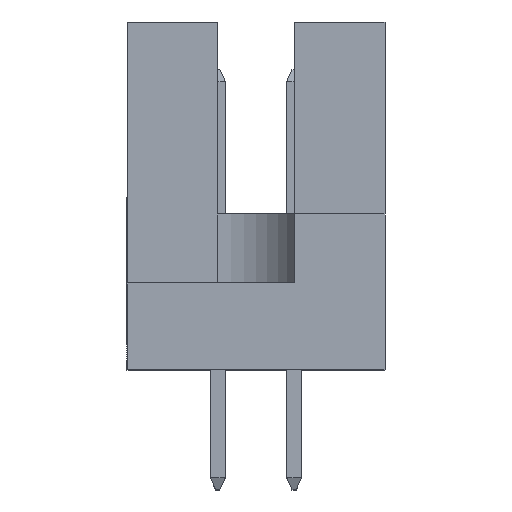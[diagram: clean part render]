
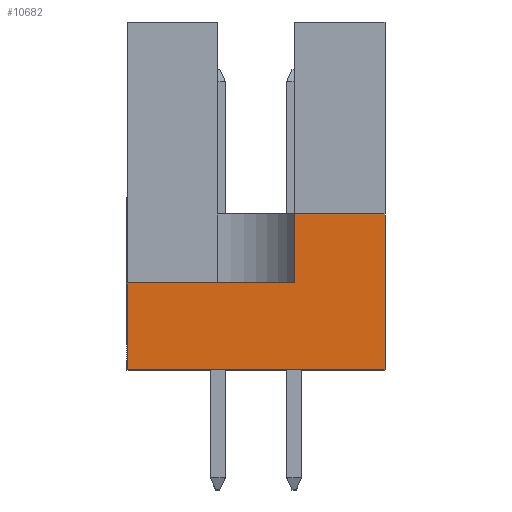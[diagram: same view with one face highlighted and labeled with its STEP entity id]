
A CAD part, left-side view. The second image highlights one B-rep face of the part: STEP entity #10682.
In plain terms, the highlighted planar face has unit normal (-1, 0, 0).
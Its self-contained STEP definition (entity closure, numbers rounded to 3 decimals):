
#444 = EDGE_CURVE ( 'NONE', #10742, #10309, #2380, .T. ) ;
#518 = VERTEX_POINT ( 'NONE', #10656 ) ;
#598 = FACE_OUTER_BOUND ( 'NONE', #5916, .T. ) ;
#908 = DIRECTION ( 'NONE',  ( 0., 0., -1. ) ) ;
#1095 = ORIENTED_EDGE ( 'NONE', *, *, #4684, .F. ) ;
#1293 = DIRECTION ( 'NONE',  ( 0., 0., -1. ) ) ;
#1471 = DIRECTION ( 'NONE',  ( 0., -1., 0. ) ) ;
#2091 = CARTESIAN_POINT ( 'NONE',  ( -47.5, 4.3, 11.6 ) ) ;
#2115 = CARTESIAN_POINT ( 'NONE',  ( -47.5, 4.3, 2.9 ) ) ;
#2380 = LINE ( 'NONE', #10337, #5114 ) ;
#2808 = VECTOR ( 'NONE', #3767, 1000. ) ;
#3012 = DIRECTION ( 'NONE',  ( 1., 0., 0. ) ) ;
#3063 = CARTESIAN_POINT ( 'NONE',  ( -47.5, 4.3, 11.6 ) ) ;
#3296 = ORIENTED_EDGE ( 'NONE', *, *, #444, .F. ) ;
#3382 = VECTOR ( 'NONE', #908, 1000. ) ;
#3767 = DIRECTION ( 'NONE',  ( 0., 0., -1. ) ) ;
#3937 = DIRECTION ( 'NONE',  ( 0., 1., 0. ) ) ;
#3950 = LINE ( 'NONE', #5848, #2808 ) ;
#3961 = LINE ( 'NONE', #3063, #3382 ) ;
#4121 = EDGE_CURVE ( 'NONE', #6215, #518, #6715, .T. ) ;
#4600 = CARTESIAN_POINT ( 'NONE',  ( -47.5, 4.3, 2.9 ) ) ;
#4615 = ORIENTED_EDGE ( 'NONE', *, *, #12720, .T. ) ;
#4631 = CARTESIAN_POINT ( 'NONE',  ( -47.5, -1.27, 2.9 ) ) ;
#4684 = EDGE_CURVE ( 'NONE', #10309, #518, #3950, .T. ) ;
#4894 = DIRECTION ( 'NONE',  ( 0., 0., -1. ) ) ;
#4970 = CARTESIAN_POINT ( 'NONE',  ( -47.5, -4.3, 5.2 ) ) ;
#5114 = VECTOR ( 'NONE', #1471, 1000. ) ;
#5848 = CARTESIAN_POINT ( 'NONE',  ( -47.5, -4.3, 11.6 ) ) ;
#5916 = EDGE_LOOP ( 'NONE', ( #3296, #4615, #6372, #6637, #11961, #1095 ) ) ;
#6215 = VERTEX_POINT ( 'NONE', #12864 ) ;
#6286 = VERTEX_POINT ( 'NONE', #4631 ) ;
#6372 = ORIENTED_EDGE ( 'NONE', *, *, #6703, .T. ) ;
#6637 = ORIENTED_EDGE ( 'NONE', *, *, #9760, .T. ) ;
#6703 = EDGE_CURVE ( 'NONE', #6286, #7880, #8896, .T. ) ;
#6715 = LINE ( 'NONE', #8537, #10976 ) ;
#7620 = VECTOR ( 'NONE', #3937, 1000. ) ;
#7880 = VERTEX_POINT ( 'NONE', #4600 ) ;
#8196 = CARTESIAN_POINT ( 'NONE',  ( -47.5, -1.27, 19.02 ) ) ;
#8537 = CARTESIAN_POINT ( 'NONE',  ( -47.5, 4.3, 0. ) ) ;
#8896 = LINE ( 'NONE', #2115, #7620 ) ;
#9760 = EDGE_CURVE ( 'NONE', #7880, #6215, #3961, .T. ) ;
#9855 = PLANE ( 'NONE',  #11312 ) ;
#10224 = LINE ( 'NONE', #8196, #10516 ) ;
#10309 = VERTEX_POINT ( 'NONE', #4970 ) ;
#10337 = CARTESIAN_POINT ( 'NONE',  ( -47.5, 4.3, 5.2 ) ) ;
#10516 = VECTOR ( 'NONE', #1293, 1000. ) ;
#10656 = CARTESIAN_POINT ( 'NONE',  ( -47.5, -4.3, 0. ) ) ;
#10682 = ADVANCED_FACE ( 'NONE', ( #598 ), #9855, .F. ) ;
#10742 = VERTEX_POINT ( 'NONE', #11962 ) ;
#10976 = VECTOR ( 'NONE', #11490, 1000. ) ;
#11312 = AXIS2_PLACEMENT_3D ( 'NONE', #2091, #3012, #4894 ) ;
#11490 = DIRECTION ( 'NONE',  ( 0., -1., 0. ) ) ;
#11961 = ORIENTED_EDGE ( 'NONE', *, *, #4121, .T. ) ;
#11962 = CARTESIAN_POINT ( 'NONE',  ( -47.5, -1.27, 5.2 ) ) ;
#12720 = EDGE_CURVE ( 'NONE', #10742, #6286, #10224, .T. ) ;
#12864 = CARTESIAN_POINT ( 'NONE',  ( -47.5, 4.3, 0. ) ) ;
